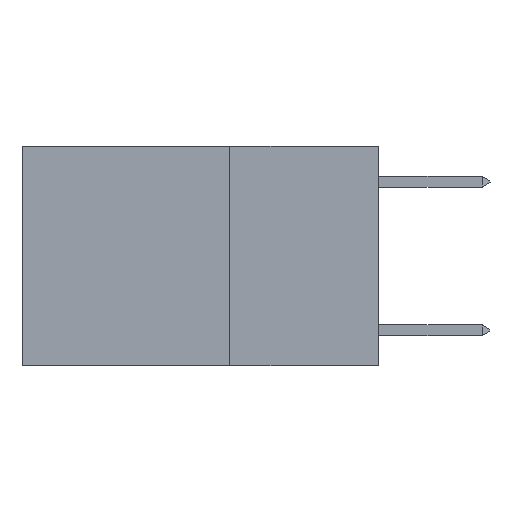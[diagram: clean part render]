
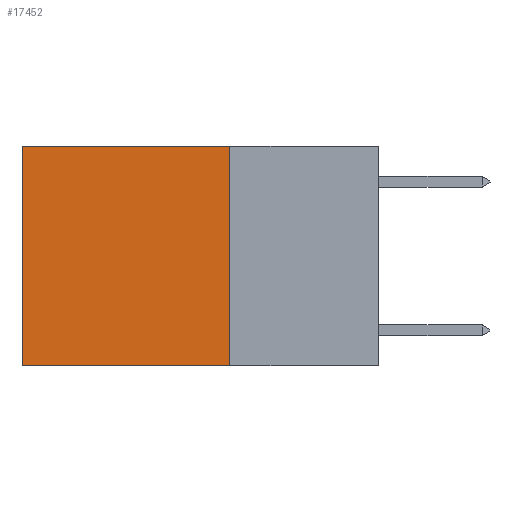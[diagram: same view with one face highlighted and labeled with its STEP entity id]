
A CAD part, left-side view. The second image highlights one B-rep face of the part: STEP entity #17452.
In plain terms, the highlighted planar face has unit normal (-1, 0, 0).
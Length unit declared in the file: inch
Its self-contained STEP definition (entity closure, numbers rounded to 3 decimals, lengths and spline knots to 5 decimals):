
#130 = LINE ( 'NONE', #2242, #24435 ) ;
#148 = EDGE_CURVE ( 'NONE', #25417, #11393, #13257, .T. ) ;
#652 = CARTESIAN_POINT ( 'NONE',  ( 0.2625, 0.25, -0.37 ) ) ;
#796 = DIRECTION ( 'NONE',  ( 0., 1., 0. ) ) ;
#1106 = DIRECTION ( 'NONE',  ( 0., 1., 0. ) ) ;
#2242 = CARTESIAN_POINT ( 'NONE',  ( 0.2625, 0.6, 0. ) ) ;
#2840 = ORIENTED_EDGE ( 'NONE', *, *, #5153, .F. ) ;
#5153 = EDGE_CURVE ( 'NONE', #11393, #29682, #21641, .T. ) ;
#6850 = DIRECTION ( 'NONE',  ( 0., 0., -1. ) ) ;
#7197 = CARTESIAN_POINT ( 'NONE',  ( 0.2625, 0.25, 0. ) ) ;
#8259 = VERTEX_POINT ( 'NONE', #17599 ) ;
#9202 = DIRECTION ( 'NONE',  ( 0., 0., -1. ) ) ;
#9339 = ORIENTED_EDGE ( 'NONE', *, *, #148, .F. ) ;
#9521 = FACE_OUTER_BOUND ( 'NONE', #13945, .T. ) ;
#11393 = VERTEX_POINT ( 'NONE', #21082 ) ;
#11675 = ORIENTED_EDGE ( 'NONE', *, *, #22187, .T. ) ;
#12368 = AXIS2_PLACEMENT_3D ( 'NONE', #21858, #28591, #19554 ) ;
#13257 = LINE ( 'NONE', #15991, #22215 ) ;
#13945 = EDGE_LOOP ( 'NONE', ( #18863, #2840, #9339, #11675 ) ) ;
#14310 = VECTOR ( 'NONE', #796, 39.37008 ) ;
#15991 = CARTESIAN_POINT ( 'NONE',  ( 0.2625, 0.25, 0. ) ) ;
#17452 = ADVANCED_FACE ( 'NONE', ( #9521 ), #26589, .F. ) ;
#17599 = CARTESIAN_POINT ( 'NONE',  ( 0.2625, 0.6, 0. ) ) ;
#18112 = CARTESIAN_POINT ( 'NONE',  ( 0.2625, 0.6, -0.37 ) ) ;
#18863 = ORIENTED_EDGE ( 'NONE', *, *, #24853, .T. ) ;
#19451 = VECTOR ( 'NONE', #1106, 39.37008 ) ;
#19554 = DIRECTION ( 'NONE',  ( 0., 0., -1. ) ) ;
#21082 = CARTESIAN_POINT ( 'NONE',  ( 0.2625, 0.25, -0.37 ) ) ;
#21641 = LINE ( 'NONE', #652, #14310 ) ;
#21679 = LINE ( 'NONE', #23964, #19451 ) ;
#21858 = CARTESIAN_POINT ( 'NONE',  ( 0.2625, 0.25, 0. ) ) ;
#22187 = EDGE_CURVE ( 'NONE', #25417, #8259, #21679, .T. ) ;
#22215 = VECTOR ( 'NONE', #6850, 39.37008 ) ;
#23964 = CARTESIAN_POINT ( 'NONE',  ( 0.2625, 0.25, 0. ) ) ;
#24435 = VECTOR ( 'NONE', #9202, 39.37008 ) ;
#24853 = EDGE_CURVE ( 'NONE', #8259, #29682, #130, .T. ) ;
#25417 = VERTEX_POINT ( 'NONE', #7197 ) ;
#26589 = PLANE ( 'NONE',  #12368 ) ;
#28591 = DIRECTION ( 'NONE',  ( 1., 0., 0. ) ) ;
#29682 = VERTEX_POINT ( 'NONE', #18112 ) ;
